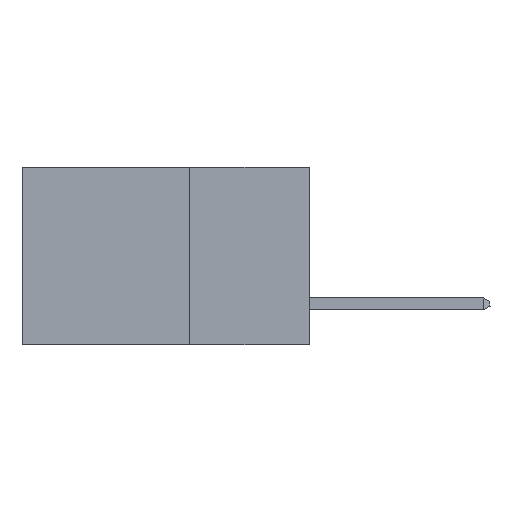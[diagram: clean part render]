
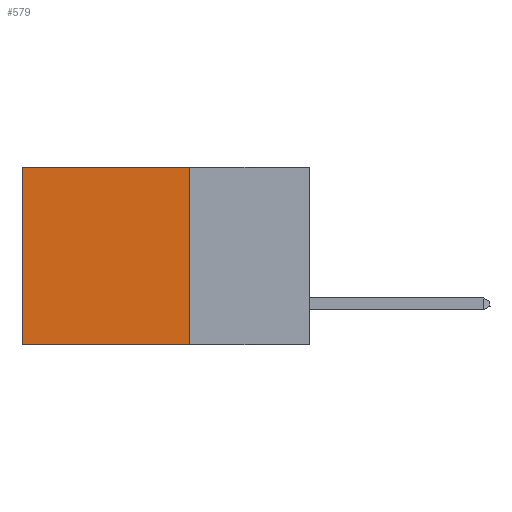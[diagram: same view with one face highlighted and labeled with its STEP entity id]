
A CAD part, left-side view. The second image highlights one B-rep face of the part: STEP entity #579.
In plain terms, the highlighted planar face has unit normal (-1, 0, 0).
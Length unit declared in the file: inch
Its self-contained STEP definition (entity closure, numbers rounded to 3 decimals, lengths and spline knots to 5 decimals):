
#579 = ADVANCED_FACE ( 'NONE', ( #13787 ), #1967, .F. ) ;
#1536 = VERTEX_POINT ( 'NONE', #8583 ) ;
#1537 = CARTESIAN_POINT ( 'NONE',  ( 0.2875, 0.6, 0. ) ) ;
#1928 = VERTEX_POINT ( 'NONE', #14621 ) ;
#1967 = PLANE ( 'NONE',  #2469 ) ;
#2469 = AXIS2_PLACEMENT_3D ( 'NONE', #5831, #7586, #9580 ) ;
#3119 = LINE ( 'NONE', #3891, #9579 ) ;
#3831 = DIRECTION ( 'NONE',  ( 0., 1., 0. ) ) ;
#3891 = CARTESIAN_POINT ( 'NONE',  ( 0.2875, 0.25, 0. ) ) ;
#3902 = VECTOR ( 'NONE', #11262, 39.37008 ) ;
#4160 = ORIENTED_EDGE ( 'NONE', *, *, #7588, .F. ) ;
#4447 = EDGE_CURVE ( 'NONE', #1928, #15240, #11114, .T. ) ;
#4748 = VERTEX_POINT ( 'NONE', #15292 ) ;
#5831 = CARTESIAN_POINT ( 'NONE',  ( 0.2875, 0.25, 0. ) ) ;
#6410 = DIRECTION ( 'NONE',  ( 0., 0., -1. ) ) ;
#6779 = DIRECTION ( 'NONE',  ( 0., 1., 0. ) ) ;
#7325 = CARTESIAN_POINT ( 'NONE',  ( 0.2875, 0.25, 0. ) ) ;
#7586 = DIRECTION ( 'NONE',  ( 1., 0., 0. ) ) ;
#7588 = EDGE_CURVE ( 'NONE', #1536, #1928, #10826, .T. ) ;
#8583 = CARTESIAN_POINT ( 'NONE',  ( 0.2875, 0.25, 0. ) ) ;
#9579 = VECTOR ( 'NONE', #3831, 39.37008 ) ;
#9580 = DIRECTION ( 'NONE',  ( 0., 0., -1. ) ) ;
#10447 = CARTESIAN_POINT ( 'NONE',  ( 0.2875, 0.6, -0.37 ) ) ;
#10826 = LINE ( 'NONE', #7325, #3902 ) ;
#11114 = LINE ( 'NONE', #15949, #16318 ) ;
#11156 = EDGE_CURVE ( 'NONE', #4748, #15240, #11466, .T. ) ;
#11262 = DIRECTION ( 'NONE',  ( 0., 0., -1. ) ) ;
#11466 = LINE ( 'NONE', #1537, #13066 ) ;
#12193 = EDGE_LOOP ( 'NONE', ( #15032, #14769, #4160, #13795 ) ) ;
#13066 = VECTOR ( 'NONE', #6410, 39.37008 ) ;
#13787 = FACE_OUTER_BOUND ( 'NONE', #12193, .T. ) ;
#13795 = ORIENTED_EDGE ( 'NONE', *, *, #16693, .T. ) ;
#14621 = CARTESIAN_POINT ( 'NONE',  ( 0.2875, 0.25, -0.37 ) ) ;
#14769 = ORIENTED_EDGE ( 'NONE', *, *, #4447, .F. ) ;
#15032 = ORIENTED_EDGE ( 'NONE', *, *, #11156, .T. ) ;
#15240 = VERTEX_POINT ( 'NONE', #10447 ) ;
#15292 = CARTESIAN_POINT ( 'NONE',  ( 0.2875, 0.6, 0. ) ) ;
#15949 = CARTESIAN_POINT ( 'NONE',  ( 0.2875, 0.25, -0.37 ) ) ;
#16318 = VECTOR ( 'NONE', #6779, 39.37008 ) ;
#16693 = EDGE_CURVE ( 'NONE', #1536, #4748, #3119, .T. ) ;
